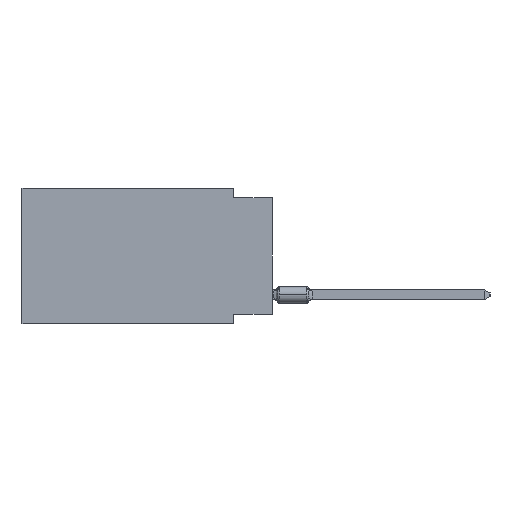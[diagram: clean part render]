
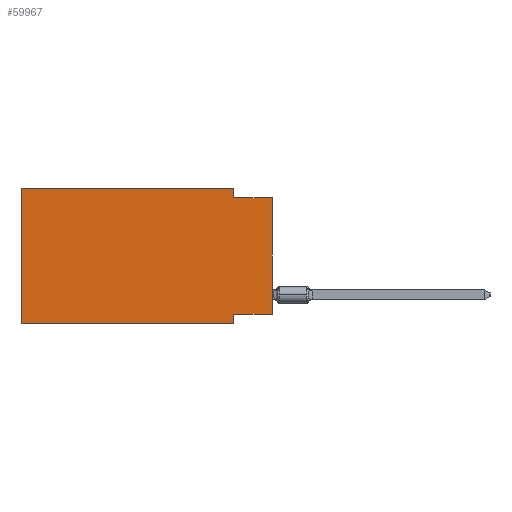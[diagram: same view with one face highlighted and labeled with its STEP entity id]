
A CAD part, left-side view. The second image highlights one B-rep face of the part: STEP entity #59967.
In plain terms, the highlighted planar face has unit normal (-1, 0, 0).
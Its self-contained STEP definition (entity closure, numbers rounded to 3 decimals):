
#518 = EDGE_CURVE ( 'NONE', #63917, #35091, #47820, .T. ) ;
#1259 = ORIENTED_EDGE ( 'NONE', *, *, #39512, .F. ) ;
#2068 = CARTESIAN_POINT ( 'NONE',  ( 0., 0., -0.635 ) ) ;
#2647 = VERTEX_POINT ( 'NONE', #31515 ) ;
#3255 = ORIENTED_EDGE ( 'NONE', *, *, #31018, .T. ) ;
#5050 = AXIS2_PLACEMENT_3D ( 'NONE', #57964, #14089, #31631 ) ;
#5519 = VERTEX_POINT ( 'NONE', #27615 ) ;
#7667 = DIRECTION ( 'NONE',  ( 0., -1., 0. ) ) ;
#7839 = DIRECTION ( 'NONE',  ( 0., -1., 0. ) ) ;
#8576 = DIRECTION ( 'NONE',  ( 0., 1., 0. ) ) ;
#9127 = VECTOR ( 'NONE', #64041, 1000. ) ;
#13064 = CARTESIAN_POINT ( 'NONE',  ( 0., 0., -8.255 ) ) ;
#13097 = CARTESIAN_POINT ( 'NONE',  ( 0., 2.54, 0. ) ) ;
#14089 = DIRECTION ( 'NONE',  ( 1., 0., 0. ) ) ;
#14704 = LINE ( 'NONE', #63817, #30250 ) ;
#19467 = ORIENTED_EDGE ( 'NONE', *, *, #66887, .F. ) ;
#20315 = DIRECTION ( 'NONE',  ( 0., 0., 1. ) ) ;
#20362 = VECTOR ( 'NONE', #30973, 1000. ) ;
#21057 = EDGE_CURVE ( 'NONE', #41657, #29603, #31766, .T. ) ;
#21536 = ORIENTED_EDGE ( 'NONE', *, *, #21057, .T. ) ;
#25061 = VERTEX_POINT ( 'NONE', #13064 ) ;
#25327 = FACE_OUTER_BOUND ( 'NONE', #52002, .T. ) ;
#25577 = CARTESIAN_POINT ( 'NONE',  ( 0., 0., -0.635 ) ) ;
#26440 = EDGE_CURVE ( 'NONE', #2647, #29603, #40883, .T. ) ;
#27615 = CARTESIAN_POINT ( 'NONE',  ( 0., 16.383, 0. ) ) ;
#28903 = CARTESIAN_POINT ( 'NONE',  ( 0., 0., 0. ) ) ;
#29603 = VERTEX_POINT ( 'NONE', #38737 ) ;
#29976 = LINE ( 'NONE', #56641, #58000 ) ;
#30250 = VECTOR ( 'NONE', #20315, 1000. ) ;
#30973 = DIRECTION ( 'NONE',  ( 0., 0., -1. ) ) ;
#31018 = EDGE_CURVE ( 'NONE', #25061, #31925, #39093, .T. ) ;
#31515 = CARTESIAN_POINT ( 'NONE',  ( 0., 2.54, -8.255 ) ) ;
#31631 = DIRECTION ( 'NONE',  ( 0., 0., -1. ) ) ;
#31766 = LINE ( 'NONE', #42651, #9127 ) ;
#31925 = VERTEX_POINT ( 'NONE', #25577 ) ;
#32995 = VECTOR ( 'NONE', #57724, 1000. ) ;
#33073 = EDGE_CURVE ( 'NONE', #41657, #5519, #14704, .T. ) ;
#33849 = EDGE_CURVE ( 'NONE', #25061, #2647, #29976, .T. ) ;
#34510 = DIRECTION ( 'NONE',  ( 0., 0., 1. ) ) ;
#34970 = ORIENTED_EDGE ( 'NONE', *, *, #33073, .F. ) ;
#35091 = VERTEX_POINT ( 'NONE', #57005 ) ;
#38737 = CARTESIAN_POINT ( 'NONE',  ( 0., 2.54, -8.89 ) ) ;
#39093 = LINE ( 'NONE', #28903, #57110 ) ;
#39512 = EDGE_CURVE ( 'NONE', #35091, #31925, #39600, .T. ) ;
#39571 = ORIENTED_EDGE ( 'NONE', *, *, #33849, .F. ) ;
#39600 = LINE ( 'NONE', #2068, #47210 ) ;
#39779 = CARTESIAN_POINT ( 'NONE',  ( 0., 16.383, 0. ) ) ;
#40883 = LINE ( 'NONE', #62273, #32995 ) ;
#41473 = PLANE ( 'NONE',  #5050 ) ;
#41657 = VERTEX_POINT ( 'NONE', #57629 ) ;
#42211 = CARTESIAN_POINT ( 'NONE',  ( 0., 2.54, 0. ) ) ;
#42651 = CARTESIAN_POINT ( 'NONE',  ( 0., 16.383, -8.89 ) ) ;
#44752 = VECTOR ( 'NONE', #7839, 1000. ) ;
#45026 = ORIENTED_EDGE ( 'NONE', *, *, #26440, .F. ) ;
#47210 = VECTOR ( 'NONE', #7667, 1000. ) ;
#47820 = LINE ( 'NONE', #42211, #20362 ) ;
#52002 = EDGE_LOOP ( 'NONE', ( #3255, #1259, #68141, #19467, #34970, #21536, #45026, #39571 ) ) ;
#56641 = CARTESIAN_POINT ( 'NONE',  ( 0., 0., -8.255 ) ) ;
#57005 = CARTESIAN_POINT ( 'NONE',  ( 0., 2.54, -0.635 ) ) ;
#57110 = VECTOR ( 'NONE', #34510, 1000. ) ;
#57629 = CARTESIAN_POINT ( 'NONE',  ( 0., 16.383, -8.89 ) ) ;
#57724 = DIRECTION ( 'NONE',  ( 0., 0., -1. ) ) ;
#57964 = CARTESIAN_POINT ( 'NONE',  ( 0., 16.383, 0. ) ) ;
#58000 = VECTOR ( 'NONE', #8576, 1000. ) ;
#59967 = ADVANCED_FACE ( 'NONE', ( #25327 ), #41473, .F. ) ;
#62273 = CARTESIAN_POINT ( 'NONE',  ( 0., 2.54, -8.89 ) ) ;
#63817 = CARTESIAN_POINT ( 'NONE',  ( 0., 16.383, 0. ) ) ;
#63917 = VERTEX_POINT ( 'NONE', #13097 ) ;
#64041 = DIRECTION ( 'NONE',  ( 0., -1., 0. ) ) ;
#66887 = EDGE_CURVE ( 'NONE', #5519, #63917, #69145, .T. ) ;
#68141 = ORIENTED_EDGE ( 'NONE', *, *, #518, .F. ) ;
#69145 = LINE ( 'NONE', #39779, #44752 ) ;
